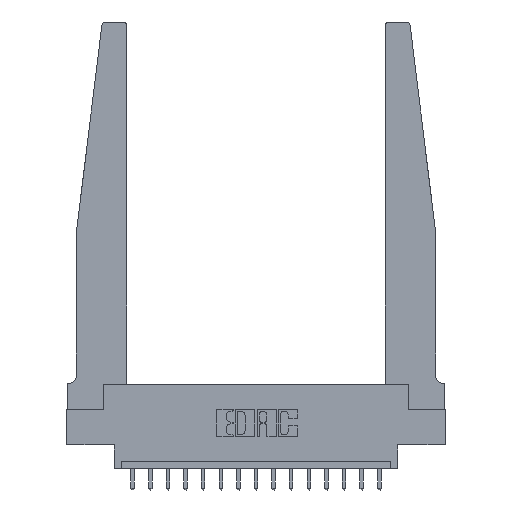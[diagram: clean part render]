
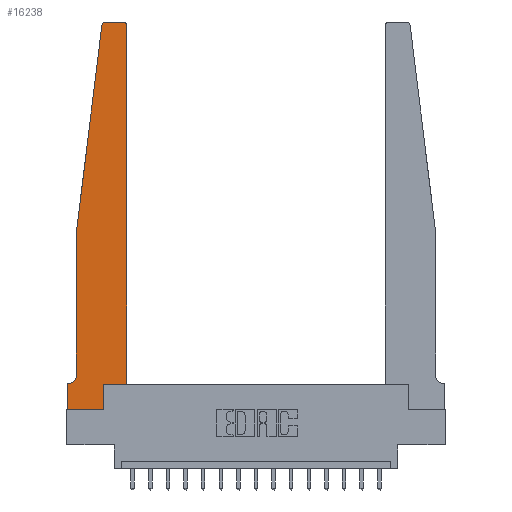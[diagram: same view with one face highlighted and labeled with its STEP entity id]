
A CAD part, top view. The second image highlights one B-rep face of the part: STEP entity #16238.
In plain terms, the highlighted planar face has unit normal (0, 0, 1).
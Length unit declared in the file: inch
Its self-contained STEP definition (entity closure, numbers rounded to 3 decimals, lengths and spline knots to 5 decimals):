
#7 = ORIENTED_EDGE ( 'NONE', *, *, #5468, .T. ) ;
#155 = VERTEX_POINT ( 'NONE', #8186 ) ;
#282 = LINE ( 'NONE', #5963, #14622 ) ;
#433 = CARTESIAN_POINT ( 'NONE',  ( 0.015, 0.1875, 0.37 ) ) ;
#959 = VECTOR ( 'NONE', #1309, 39.37008 ) ;
#1065 = EDGE_CURVE ( 'NONE', #1784, #10791, #11406, .T. ) ;
#1099 = CARTESIAN_POINT ( 'NONE',  ( 0., 0.1875, 0.37 ) ) ;
#1309 = DIRECTION ( 'NONE',  ( 0., 1., 0. ) ) ;
#1400 = CARTESIAN_POINT ( 'NONE',  ( 0.425, 0.18, 0.37 ) ) ;
#1450 = ORIENTED_EDGE ( 'NONE', *, *, #8248, .T. ) ;
#1492 = ORIENTED_EDGE ( 'NONE', *, *, #7028, .T. ) ;
#1514 = ORIENTED_EDGE ( 'NONE', *, *, #11915, .T. ) ;
#1575 = VERTEX_POINT ( 'NONE', #433 ) ;
#1784 = VERTEX_POINT ( 'NONE', #16708 ) ;
#2249 = CARTESIAN_POINT ( 'NONE',  ( 0.2605, 0., 0.37 ) ) ;
#2647 = LINE ( 'NONE', #8407, #11160 ) ;
#2759 = DIRECTION ( 'NONE',  ( 1., 0., 0. ) ) ;
#3203 = DIRECTION ( 'NONE',  ( -1., 0., 0. ) ) ;
#3482 = VECTOR ( 'NONE', #14022, 39.37008 ) ;
#3748 = CARTESIAN_POINT ( 'NONE',  ( 0.27653, 2.75, 0.37 ) ) ;
#4172 = VECTOR ( 'NONE', #15645, 39.37008 ) ;
#4322 = ORIENTED_EDGE ( 'NONE', *, *, #5107, .T. ) ;
#4504 = CARTESIAN_POINT ( 'NONE',  ( 0.065, 1.25, 0.37 ) ) ;
#4828 = EDGE_CURVE ( 'NONE', #7707, #14363, #12888, .T. ) ;
#4847 = EDGE_CURVE ( 'NONE', #16163, #1784, #282, .T. ) ;
#5075 = ORIENTED_EDGE ( 'NONE', *, *, #1065, .T. ) ;
#5105 = CARTESIAN_POINT ( 'NONE',  ( 0.395, 2.72, 0.37 ) ) ;
#5107 = EDGE_CURVE ( 'NONE', #7546, #13972, #2647, .T. ) ;
#5146 = CARTESIAN_POINT ( 'NONE',  ( 0., 0.1875, 0.37 ) ) ;
#5213 = EDGE_CURVE ( 'NONE', #155, #15512, #14402, .T. ) ;
#5405 = DIRECTION ( 'NONE',  ( 1., 0., 0. ) ) ;
#5438 = LINE ( 'NONE', #11167, #3482 ) ;
#5468 = EDGE_CURVE ( 'NONE', #14328, #16163, #5438, .T. ) ;
#5703 = ORIENTED_EDGE ( 'NONE', *, *, #4847, .T. ) ;
#5841 = CARTESIAN_POINT ( 'NONE',  ( 0.015, 0.2375, 0.37 ) ) ;
#5865 = DIRECTION ( 'NONE',  ( 0., -1., 0. ) ) ;
#5963 = CARTESIAN_POINT ( 'NONE',  ( 0.425, 0.18, 0.37 ) ) ;
#6685 = ORIENTED_EDGE ( 'NONE', *, *, #5213, .T. ) ;
#6699 = PLANE ( 'NONE',  #8856 ) ;
#6831 = DIRECTION ( 'NONE',  ( 0., 0., 1. ) ) ;
#7004 = CARTESIAN_POINT ( 'NONE',  ( 0.065, 1.25, 0.37 ) ) ;
#7012 = CIRCLE ( 'NONE', #15542, 0.05 ) ;
#7028 = EDGE_CURVE ( 'NONE', #13972, #17493, #8454, .T. ) ;
#7198 = ORIENTED_EDGE ( 'NONE', *, *, #8692, .T. ) ;
#7458 = CARTESIAN_POINT ( 'NONE',  ( 0.27653, 2.72, 0.37 ) ) ;
#7546 = VERTEX_POINT ( 'NONE', #14798 ) ;
#7707 = VERTEX_POINT ( 'NONE', #1099 ) ;
#7935 = DIRECTION ( 'NONE',  ( 1., 0., 0. ) ) ;
#8186 = CARTESIAN_POINT ( 'NONE',  ( 0.395, 2.75, 0.37 ) ) ;
#8248 = EDGE_CURVE ( 'NONE', #15512, #7546, #10100, .T. ) ;
#8407 = CARTESIAN_POINT ( 'NONE',  ( 0.065, 1.25, 0.37 ) ) ;
#8454 = LINE ( 'NONE', #4504, #4172 ) ;
#8631 = CARTESIAN_POINT ( 'NONE',  ( 0., 0., 0.37 ) ) ;
#8692 = EDGE_CURVE ( 'NONE', #1575, #7707, #11051, .T. ) ;
#8856 = AXIS2_PLACEMENT_3D ( 'NONE', #5146, #12337, #5405 ) ;
#8963 = VECTOR ( 'NONE', #15258, 39.37008 ) ;
#10100 = CIRCLE ( 'NONE', #11881, 0.03 ) ;
#10568 = AXIS2_PLACEMENT_3D ( 'NONE', #5105, #6831, #7935 ) ;
#10585 = EDGE_CURVE ( 'NONE', #14363, #14328, #14044, .T. ) ;
#10773 = CARTESIAN_POINT ( 'NONE',  ( 0.065, 0.2375, 0.37 ) ) ;
#10791 = VERTEX_POINT ( 'NONE', #14498 ) ;
#11051 = LINE ( 'NONE', #16858, #8963 ) ;
#11160 = VECTOR ( 'NONE', #11287, 39.37008 ) ;
#11167 = CARTESIAN_POINT ( 'NONE',  ( 0.2605, 0.18, 0.37 ) ) ;
#11287 = DIRECTION ( 'NONE',  ( -0.122, -0.992, 0. ) ) ;
#11406 = LINE ( 'NONE', #1400, #959 ) ;
#11450 = VECTOR ( 'NONE', #3203, 39.37008 ) ;
#11672 = ORIENTED_EDGE ( 'NONE', *, *, #4828, .T. ) ;
#11881 = AXIS2_PLACEMENT_3D ( 'NONE', #7458, #13188, #15854 ) ;
#11915 = EDGE_CURVE ( 'NONE', #17493, #1575, #7012, .T. ) ;
#12159 = EDGE_CURVE ( 'NONE', #10791, #155, #17929, .T. ) ;
#12337 = DIRECTION ( 'NONE',  ( 0., 0., 1. ) ) ;
#12888 = LINE ( 'NONE', #8631, #16980 ) ;
#13188 = DIRECTION ( 'NONE',  ( 0., 0., 1. ) ) ;
#13219 = DIRECTION ( 'NONE',  ( 0., 0., -1. ) ) ;
#13720 = FACE_OUTER_BOUND ( 'NONE', #16746, .T. ) ;
#13972 = VERTEX_POINT ( 'NONE', #7004 ) ;
#14022 = DIRECTION ( 'NONE',  ( 0., 1., 0. ) ) ;
#14044 = LINE ( 'NONE', #16634, #14435 ) ;
#14328 = VERTEX_POINT ( 'NONE', #2249 ) ;
#14363 = VERTEX_POINT ( 'NONE', #17787 ) ;
#14402 = LINE ( 'NONE', #15876, #11450 ) ;
#14435 = VECTOR ( 'NONE', #2759, 39.37008 ) ;
#14498 = CARTESIAN_POINT ( 'NONE',  ( 0.425, 2.72, 0.37 ) ) ;
#14567 = ORIENTED_EDGE ( 'NONE', *, *, #10585, .T. ) ;
#14622 = VECTOR ( 'NONE', #16757, 39.37008 ) ;
#14798 = CARTESIAN_POINT ( 'NONE',  ( 0.24675, 2.72367, 0.37 ) ) ;
#14992 = CARTESIAN_POINT ( 'NONE',  ( 0.2605, 0.18, 0.37 ) ) ;
#15258 = DIRECTION ( 'NONE',  ( -1., 0., 0. ) ) ;
#15512 = VERTEX_POINT ( 'NONE', #3748 ) ;
#15542 = AXIS2_PLACEMENT_3D ( 'NONE', #5841, #13219, #17641 ) ;
#15645 = DIRECTION ( 'NONE',  ( 0., -1., 0. ) ) ;
#15854 = DIRECTION ( 'NONE',  ( 1., 0., 0. ) ) ;
#15876 = CARTESIAN_POINT ( 'NONE',  ( 0.25, 2.75, 0.37 ) ) ;
#16163 = VERTEX_POINT ( 'NONE', #14992 ) ;
#16238 = ADVANCED_FACE ( 'NONE', ( #13720 ), #6699, .T. ) ;
#16634 = CARTESIAN_POINT ( 'NONE',  ( 0., 0., 0.37 ) ) ;
#16708 = CARTESIAN_POINT ( 'NONE',  ( 0.425, 0.18, 0.37 ) ) ;
#16746 = EDGE_LOOP ( 'NONE', ( #6685, #1450, #4322, #1492, #1514, #7198, #11672, #14567, #7, #5703, #5075, #17910 ) ) ;
#16757 = DIRECTION ( 'NONE',  ( 1., 0., 0. ) ) ;
#16858 = CARTESIAN_POINT ( 'NONE',  ( 0.065, 0.1875, 0.37 ) ) ;
#16980 = VECTOR ( 'NONE', #5865, 39.37008 ) ;
#17493 = VERTEX_POINT ( 'NONE', #10773 ) ;
#17641 = DIRECTION ( 'NONE',  ( -1., 0., 0. ) ) ;
#17787 = CARTESIAN_POINT ( 'NONE',  ( 0., 0., 0.37 ) ) ;
#17910 = ORIENTED_EDGE ( 'NONE', *, *, #12159, .T. ) ;
#17929 = CIRCLE ( 'NONE', #10568, 0.03 ) ;
